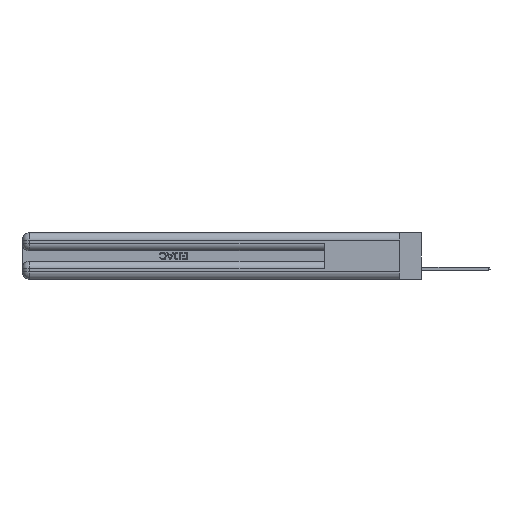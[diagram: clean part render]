
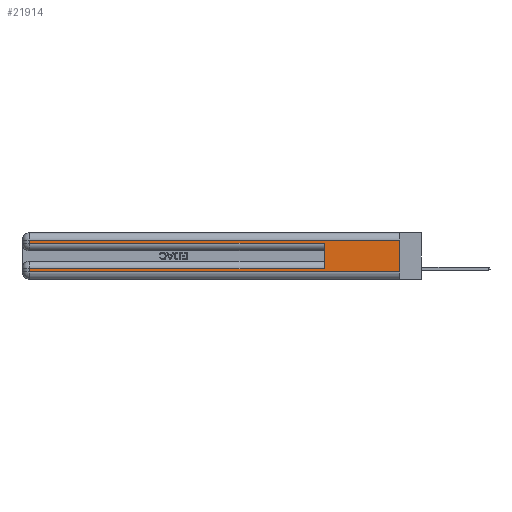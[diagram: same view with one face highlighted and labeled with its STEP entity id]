
A CAD part, left-side view. The second image highlights one B-rep face of the part: STEP entity #21914.
In plain terms, the highlighted planar face has unit normal (-1, 0, 0).
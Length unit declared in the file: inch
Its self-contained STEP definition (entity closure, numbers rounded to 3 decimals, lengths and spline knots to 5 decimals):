
#896 = VERTEX_POINT ( 'NONE', #50328 ) ;
#1808 = EDGE_CURVE ( 'NONE', #35663, #45432, #31153, .T. ) ;
#2222 = DIRECTION ( 'NONE',  ( 0., -1., 0. ) ) ;
#2409 = EDGE_CURVE ( 'NONE', #40392, #7072, #48125, .T. ) ;
#2465 = VECTOR ( 'NONE', #49197, 39.37008 ) ;
#2483 = EDGE_CURVE ( 'NONE', #44973, #44279, #12811, .T. ) ;
#2894 = LINE ( 'NONE', #5614, #44312 ) ;
#3009 = DIRECTION ( 'NONE',  ( 1., 0., 0. ) ) ;
#3222 = CARTESIAN_POINT ( 'NONE',  ( 0., 2.94, 0.085 ) ) ;
#3694 = CARTESIAN_POINT ( 'NONE',  ( 0., 0., 0.37 ) ) ;
#5327 = EDGE_CURVE ( 'NONE', #896, #45432, #2894, .T. ) ;
#5614 = CARTESIAN_POINT ( 'NONE',  ( 0., 0.6, 0.145 ) ) ;
#7023 = CARTESIAN_POINT ( 'NONE',  ( 0., 0., 0.285 ) ) ;
#7072 = VERTEX_POINT ( 'NONE', #21432 ) ;
#7392 = ORIENTED_EDGE ( 'NONE', *, *, #47401, .T. ) ;
#7424 = LINE ( 'NONE', #37299, #2465 ) ;
#7820 = CARTESIAN_POINT ( 'NONE',  ( 0., 0., 0.06 ) ) ;
#9248 = ORIENTED_EDGE ( 'NONE', *, *, #2409, .T. ) ;
#9369 = CARTESIAN_POINT ( 'NONE',  ( 0., 0., 0.31 ) ) ;
#12304 = LINE ( 'NONE', #23628, #46424 ) ;
#12811 = LINE ( 'NONE', #7820, #45168 ) ;
#14940 = CARTESIAN_POINT ( 'NONE',  ( 0., 0.6, 0.285 ) ) ;
#16976 = FACE_OUTER_BOUND ( 'NONE', #39390, .T. ) ;
#17415 = DIRECTION ( 'NONE',  ( 0., 0., -1. ) ) ;
#20705 = VECTOR ( 'NONE', #26591, 39.37008 ) ;
#21432 = CARTESIAN_POINT ( 'NONE',  ( 0., 2.94, 0.31 ) ) ;
#21823 = CARTESIAN_POINT ( 'NONE',  ( 0., 2.94, 0.285 ) ) ;
#21914 = ADVANCED_FACE ( 'NONE', ( #16976 ), #26554, .F. ) ;
#22905 = ORIENTED_EDGE ( 'NONE', *, *, #5327, .F. ) ;
#23265 = VECTOR ( 'NONE', #17415, 39.37008 ) ;
#23628 = CARTESIAN_POINT ( 'NONE',  ( 0., 0., 0.085 ) ) ;
#24293 = EDGE_CURVE ( 'NONE', #7072, #35663, #7424, .T. ) ;
#24736 = EDGE_CURVE ( 'NONE', #40392, #44279, #45746, .T. ) ;
#26075 = ORIENTED_EDGE ( 'NONE', *, *, #42680, .T. ) ;
#26554 = PLANE ( 'NONE',  #42960 ) ;
#26591 = DIRECTION ( 'NONE',  ( 0., -1., 0. ) ) ;
#28967 = CARTESIAN_POINT ( 'NONE',  ( 0., 0., 0.37 ) ) ;
#29980 = LINE ( 'NONE', #40196, #23265 ) ;
#30116 = VERTEX_POINT ( 'NONE', #3222 ) ;
#30312 = DIRECTION ( 'NONE',  ( 0., 0., -1. ) ) ;
#31153 = LINE ( 'NONE', #7023, #20705 ) ;
#31154 = DIRECTION ( 'NONE',  ( 0., 1., 0. ) ) ;
#35355 = VECTOR ( 'NONE', #45121, 39.37008 ) ;
#35663 = VERTEX_POINT ( 'NONE', #21823 ) ;
#36727 = ORIENTED_EDGE ( 'NONE', *, *, #2483, .T. ) ;
#37299 = CARTESIAN_POINT ( 'NONE',  ( 0., 2.94, 0.37 ) ) ;
#37526 = ORIENTED_EDGE ( 'NONE', *, *, #24736, .F. ) ;
#39390 = EDGE_LOOP ( 'NONE', ( #37526, #9248, #45374, #45351, #22905, #7392, #26075, #36727 ) ) ;
#40196 = CARTESIAN_POINT ( 'NONE',  ( 0., 2.94, 0.37 ) ) ;
#40392 = VERTEX_POINT ( 'NONE', #9369 ) ;
#40859 = DIRECTION ( 'NONE',  ( 0., 0., -1. ) ) ;
#41173 = CARTESIAN_POINT ( 'NONE',  ( 0., 0., 0.31 ) ) ;
#42680 = EDGE_CURVE ( 'NONE', #30116, #44973, #29980, .T. ) ;
#42960 = AXIS2_PLACEMENT_3D ( 'NONE', #3694, #3009, #30312 ) ;
#44279 = VERTEX_POINT ( 'NONE', #47470 ) ;
#44312 = VECTOR ( 'NONE', #49216, 39.37008 ) ;
#44973 = VERTEX_POINT ( 'NONE', #46833 ) ;
#45121 = DIRECTION ( 'NONE',  ( 0., 1., 0. ) ) ;
#45168 = VECTOR ( 'NONE', #2222, 39.37008 ) ;
#45351 = ORIENTED_EDGE ( 'NONE', *, *, #1808, .T. ) ;
#45374 = ORIENTED_EDGE ( 'NONE', *, *, #24293, .T. ) ;
#45432 = VERTEX_POINT ( 'NONE', #14940 ) ;
#45746 = LINE ( 'NONE', #28967, #46936 ) ;
#46424 = VECTOR ( 'NONE', #31154, 39.37008 ) ;
#46833 = CARTESIAN_POINT ( 'NONE',  ( 0., 2.94, 0.06 ) ) ;
#46936 = VECTOR ( 'NONE', #40859, 39.37008 ) ;
#47401 = EDGE_CURVE ( 'NONE', #896, #30116, #12304, .T. ) ;
#47470 = CARTESIAN_POINT ( 'NONE',  ( 0., 0., 0.06 ) ) ;
#48125 = LINE ( 'NONE', #41173, #35355 ) ;
#49197 = DIRECTION ( 'NONE',  ( 0., 0., -1. ) ) ;
#49216 = DIRECTION ( 'NONE',  ( 0., 0., 1. ) ) ;
#50328 = CARTESIAN_POINT ( 'NONE',  ( 0., 0.6, 0.085 ) ) ;
